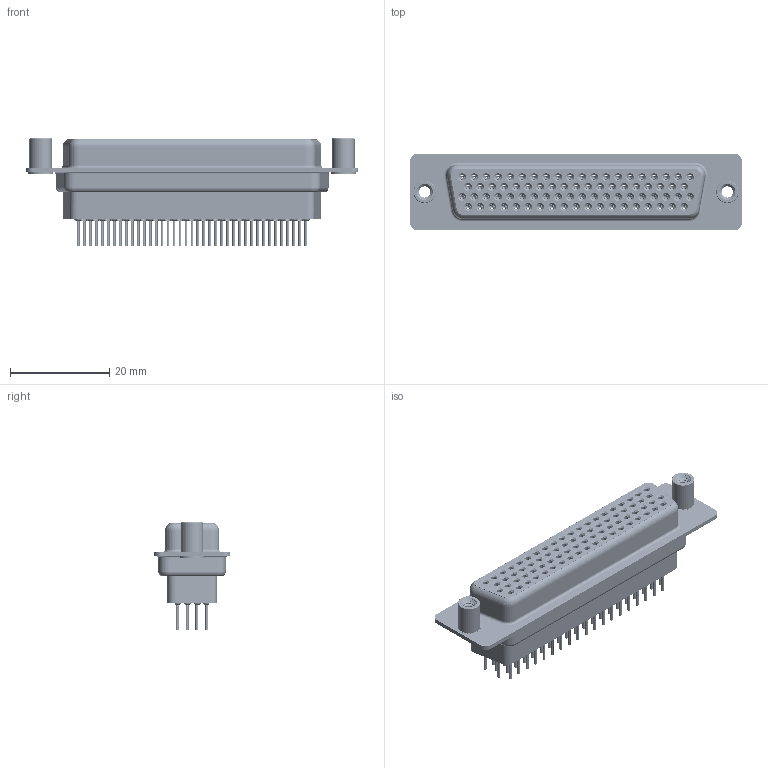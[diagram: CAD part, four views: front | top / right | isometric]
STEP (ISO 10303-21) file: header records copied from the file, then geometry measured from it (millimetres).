
FILE_DESCRIPTION (( 'STEP AP203' ), '1' );
FILE_NAME ('638-078-631-078.STEP', '2020-07-20T04:50:06', ( '' ), ( '' ), 'SwSTEP 2.0', 'SolidWorks 2020', '' );
FILE_SCHEMA (( 'CONFIG_CONTROL_DESIGN' ));
Length unit declared in the file: millimetre
Products named in the file (9): 638 Shell Rear_78 Contacts; 638 Contact Row 78_31; 638 Contact Row 3_31; 638 Shell Front_78 Contacts; 638 4-40 Threaded Standoff; 638 Contact Row 1_31; 638-078-631-078; 638 Contact Row 2_31; 638 Housing_78 Contacts HP
Assembly tree (83 placements, depth 2):
  638-078-631-078
    638 Housing_78 Contacts HP
    638 Shell Front_78 Contacts
    638 Shell Rear_78 Contacts
    638 Contact Row 1_31  x19
    638 Contact Row 2_31  x20
    638 Contact Row 3_31  x19
    638 Contact Row 78_31  x20
    638 4-40 Threaded Standoff  x2
Bounding box: 67 x 15.4 x 21.7 mm (x, y, z)
Volume: 7372.5 mm3; surface area: 25206.6 mm2
Topology: 83 solids, 83 shells, 9907 faces, 25425 edges, 15853 vertices
Faces by surface type: cylinder 2739, plane 2487, torus 1929, bspline 1566, cone 1186
Entity records: 58292 total; most frequent: CARTESIAN_POINT 14980, DIRECTION 9038, ORIENTED_EDGE 7964, EDGE_CURVE 3982, AXIS2_PLACEMENT_3D 3825, VERTEX_POINT 2525, EDGE_LOOP 2131, CIRCLE 2105
